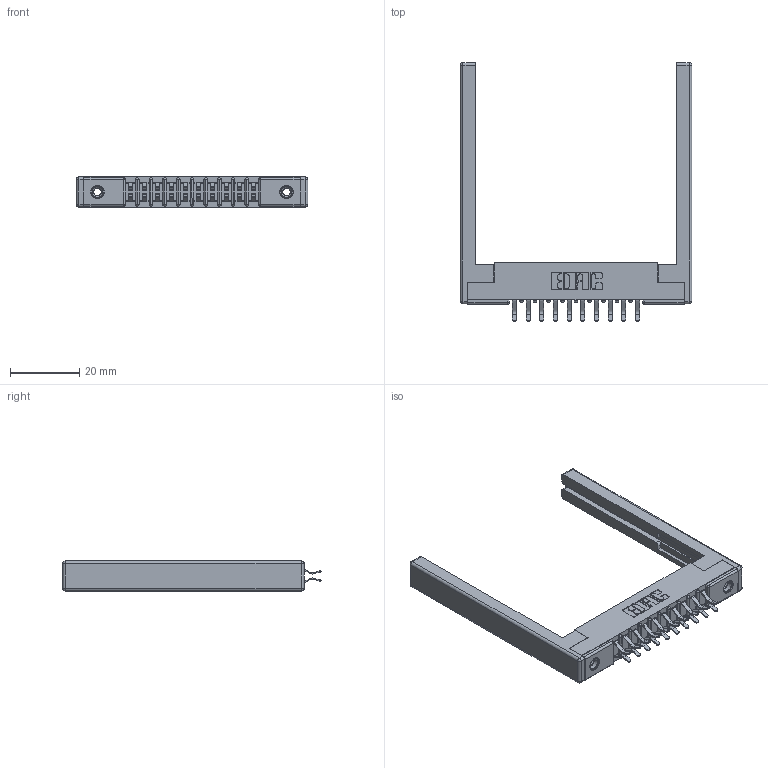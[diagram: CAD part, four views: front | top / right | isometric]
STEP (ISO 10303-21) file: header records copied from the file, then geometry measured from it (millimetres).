
FILE_DESCRIPTION (( 'STEP AP203' ), '1' );
FILE_NAME ('307-020-456-268.STEP', '2020-09-28T20:35:21', ( '' ), ( '' ), 'SwSTEP 2.0', 'SolidWorks 2020', '' );
FILE_SCHEMA (( 'CONFIG_CONTROL_DESIGN' ));
Length unit declared in the file: inch
Products named in the file (5): 307 Part_.156 Dia Mounting Holes; 307-290-001_556; 345-250-001_345-250-001-102; 307-220-068; 307-020-456-268
Assembly tree (25 placements, depth 2):
  307-020-456-268
    307 Part_.156 Dia Mounting Holes
    307-290-001_556  x20
    307-220-068  x2
    345-250-001_345-250-001-102  x2
Bounding box: 67.06 x 74.93 x 8.71 mm (x, y, z)
Volume: 8945.4 mm3; surface area: 11141.2 mm2
Topology: 25 solids, 25 shells, 1283 faces, 3553 edges, 2290 vertices
Faces by surface type: plane 818, cylinder 419, sphere 30, cone 12, torus 4
Entity records: 15701 total; most frequent: CARTESIAN_POINT 2555, DIRECTION 2532, ORIENTED_EDGE 2520, EDGE_CURVE 1260, VECTOR 950, LINE 950, VERTEX_POINT 814, AXIS2_PLACEMENT_3D 791
